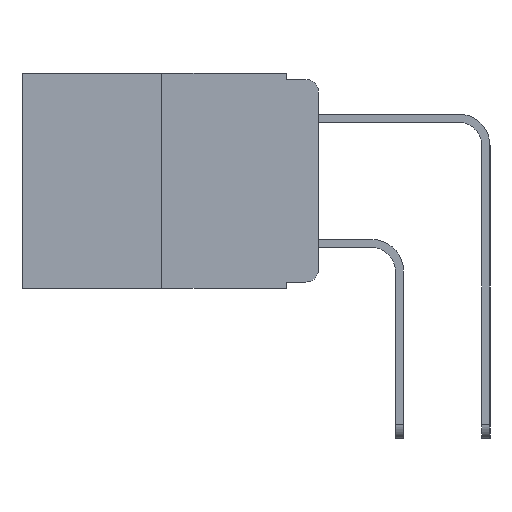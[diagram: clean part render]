
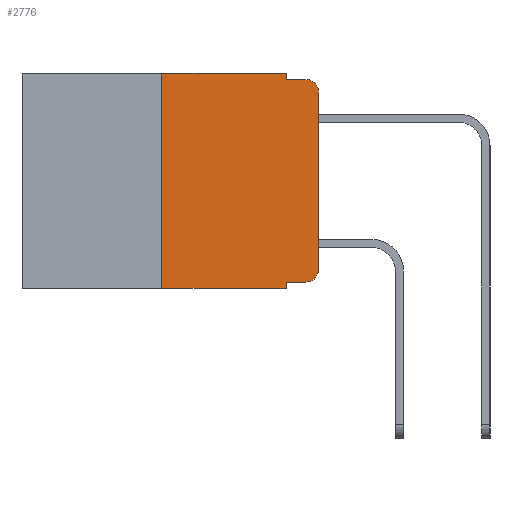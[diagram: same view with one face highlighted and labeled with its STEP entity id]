
A CAD part, left-side view. The second image highlights one B-rep face of the part: STEP entity #2776.
In plain terms, the highlighted planar face has unit normal (-1, 0, 0).
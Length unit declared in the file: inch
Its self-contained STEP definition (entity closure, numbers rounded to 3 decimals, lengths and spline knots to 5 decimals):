
#137 = LINE ( 'NONE', #9743, #8701 ) ;
#511 = VERTEX_POINT ( 'NONE', #7626 ) ;
#577 = EDGE_CURVE ( 'NONE', #13510, #2017, #5303, .T. ) ;
#598 = CARTESIAN_POINT ( 'NONE',  ( 0., 0.473, -0.343 ) ) ;
#604 = CIRCLE ( 'NONE', #8874, 0.02 ) ;
#787 = EDGE_CURVE ( 'NONE', #6568, #1679, #4307, .T. ) ;
#809 = EDGE_CURVE ( 'NONE', #1679, #13153, #604, .T. ) ;
#812 = EDGE_CURVE ( 'NONE', #6381, #13153, #137, .T. ) ;
#813 = EDGE_CURVE ( 'NONE', #511, #6381, #6382, .T. ) ;
#839 = EDGE_CURVE ( 'NONE', #13510, #10500, #2873, .T. ) ;
#841 = EDGE_CURVE ( 'NONE', #13011, #2017, #10639, .T. ) ;
#843 = EDGE_CURVE ( 'NONE', #13011, #13256, #5434, .T. ) ;
#865 = EDGE_CURVE ( 'NONE', #13256, #6568, #7780, .T. ) ;
#934 = DIRECTION ( 'NONE',  ( 0., -1., 0. ) ) ;
#1048 = VECTOR ( 'NONE', #2229, 39.37008 ) ;
#1284 = CARTESIAN_POINT ( 'NONE',  ( 0., 0.051, -0.343 ) ) ;
#1371 = CARTESIAN_POINT ( 'NONE',  ( 0., 0.051, -0.333 ) ) ;
#1487 = DIRECTION ( 'NONE',  ( 1., 0., 0. ) ) ;
#1566 = CARTESIAN_POINT ( 'NONE',  ( 0., 0.02, -0.01 ) ) ;
#1679 = VERTEX_POINT ( 'NONE', #12091 ) ;
#2012 = CARTESIAN_POINT ( 'NONE',  ( 0., 0.25, 0. ) ) ;
#2017 = VERTEX_POINT ( 'NONE', #1284 ) ;
#2229 = DIRECTION ( 'NONE',  ( 0., 0., 1. ) ) ;
#2468 = VECTOR ( 'NONE', #7109, 39.37008 ) ;
#2702 = VECTOR ( 'NONE', #8228, 39.37008 ) ;
#2776 = ADVANCED_FACE ( 'NONE', ( #13102 ), #4971, .F. ) ;
#2873 = LINE ( 'NONE', #2012, #13168 ) ;
#3250 = VECTOR ( 'NONE', #4271, 39.37008 ) ;
#3377 = DIRECTION ( 'NONE',  ( 0., -1., 0. ) ) ;
#3466 = CARTESIAN_POINT ( 'NONE',  ( 0., 0., 0. ) ) ;
#3676 = DIRECTION ( 'NONE',  ( 0., -1., 0. ) ) ;
#3768 = CARTESIAN_POINT ( 'NONE',  ( 0., 0.051, 0. ) ) ;
#3984 = ORIENTED_EDGE ( 'NONE', *, *, #787, .T. ) ;
#4130 = ORIENTED_EDGE ( 'NONE', *, *, #809, .T. ) ;
#4193 = ORIENTED_EDGE ( 'NONE', *, *, #812, .F. ) ;
#4271 = DIRECTION ( 'NONE',  ( 0., 0., -1. ) ) ;
#4273 = ORIENTED_EDGE ( 'NONE', *, *, #813, .F. ) ;
#4307 = LINE ( 'NONE', #3466, #1048 ) ;
#4358 = ORIENTED_EDGE ( 'NONE', *, *, #10511, .F. ) ;
#4378 = ORIENTED_EDGE ( 'NONE', *, *, #839, .F. ) ;
#4458 = ORIENTED_EDGE ( 'NONE', *, *, #577, .T. ) ;
#4483 = ORIENTED_EDGE ( 'NONE', *, *, #841, .F. ) ;
#4532 = ORIENTED_EDGE ( 'NONE', *, *, #843, .T. ) ;
#4563 = ORIENTED_EDGE ( 'NONE', *, *, #865, .T. ) ;
#4859 = CARTESIAN_POINT ( 'NONE',  ( 0., 0.02, -0.313 ) ) ;
#4971 = PLANE ( 'NONE',  #12666 ) ;
#4998 = DIRECTION ( 'NONE',  ( 0., 0., 1. ) ) ;
#5156 = CARTESIAN_POINT ( 'NONE',  ( 0., 0.02, -0.333 ) ) ;
#5303 = LINE ( 'NONE', #598, #7640 ) ;
#5434 = LINE ( 'NONE', #7095, #10331 ) ;
#5621 = LINE ( 'NONE', #13005, #2702 ) ;
#6381 = VERTEX_POINT ( 'NONE', #9398 ) ;
#6382 = LINE ( 'NONE', #11316, #3250 ) ;
#6435 = DIRECTION ( 'NONE',  ( 0., 0., -1. ) ) ;
#6568 = VERTEX_POINT ( 'NONE', #11423 ) ;
#7095 = CARTESIAN_POINT ( 'NONE',  ( 0., 0.051, -0.333 ) ) ;
#7109 = DIRECTION ( 'NONE',  ( 0., 0., -1. ) ) ;
#7374 = DIRECTION ( 'NONE',  ( -1., 0., 0. ) ) ;
#7626 = CARTESIAN_POINT ( 'NONE',  ( 0., 0.051, 0. ) ) ;
#7640 = VECTOR ( 'NONE', #934, 39.37008 ) ;
#7780 = CIRCLE ( 'NONE', #12079, 0.02 ) ;
#7997 = CARTESIAN_POINT ( 'NONE',  ( 0., 0.473, 0. ) ) ;
#8228 = DIRECTION ( 'NONE',  ( 0., -1., 0. ) ) ;
#8380 = CARTESIAN_POINT ( 'NONE',  ( 0., 0.25, -0.343 ) ) ;
#8701 = VECTOR ( 'NONE', #3377, 39.37008 ) ;
#8874 = AXIS2_PLACEMENT_3D ( 'NONE', #9793, #9182, #9247 ) ;
#8984 = DIRECTION ( 'NONE',  ( 0., 0., -1. ) ) ;
#9182 = DIRECTION ( 'NONE',  ( -1., 0., 0. ) ) ;
#9247 = DIRECTION ( 'NONE',  ( 0., 0., -1. ) ) ;
#9398 = CARTESIAN_POINT ( 'NONE',  ( 0., 0.051, -0.01 ) ) ;
#9743 = CARTESIAN_POINT ( 'NONE',  ( 0., 0.051, -0.01 ) ) ;
#9793 = CARTESIAN_POINT ( 'NONE',  ( 0., 0.02, -0.03 ) ) ;
#10331 = VECTOR ( 'NONE', #3676, 39.37008 ) ;
#10500 = VERTEX_POINT ( 'NONE', #11073 ) ;
#10511 = EDGE_CURVE ( 'NONE', #10500, #511, #5621, .T. ) ;
#10639 = LINE ( 'NONE', #3768, #2468 ) ;
#11073 = CARTESIAN_POINT ( 'NONE',  ( 0., 0.25, 0. ) ) ;
#11316 = CARTESIAN_POINT ( 'NONE',  ( 0., 0.051, 0. ) ) ;
#11423 = CARTESIAN_POINT ( 'NONE',  ( 0., 0., -0.313 ) ) ;
#12079 = AXIS2_PLACEMENT_3D ( 'NONE', #4859, #7374, #6435 ) ;
#12091 = CARTESIAN_POINT ( 'NONE',  ( 0., 0., -0.03 ) ) ;
#12666 = AXIS2_PLACEMENT_3D ( 'NONE', #7997, #1487, #8984 ) ;
#13005 = CARTESIAN_POINT ( 'NONE',  ( 0., 0.473, 0. ) ) ;
#13011 = VERTEX_POINT ( 'NONE', #1371 ) ;
#13102 = FACE_OUTER_BOUND ( 'NONE', #13284, .T. ) ;
#13153 = VERTEX_POINT ( 'NONE', #1566 ) ;
#13168 = VECTOR ( 'NONE', #4998, 39.37008 ) ;
#13256 = VERTEX_POINT ( 'NONE', #5156 ) ;
#13284 = EDGE_LOOP ( 'NONE', ( #3984, #4130, #4193, #4273, #4358, #4378, #4458, #4483, #4532, #4563 ) ) ;
#13510 = VERTEX_POINT ( 'NONE', #8380 ) ;
